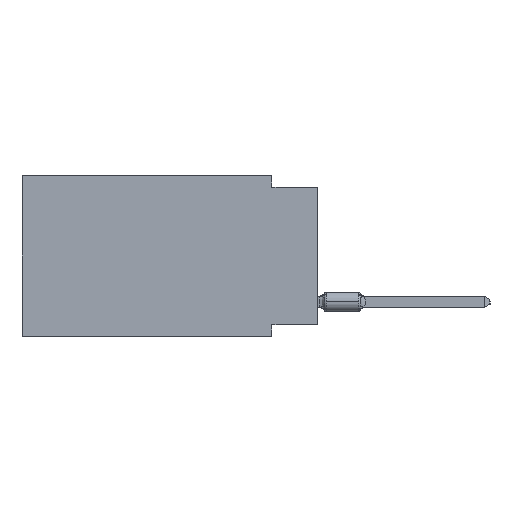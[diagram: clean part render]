
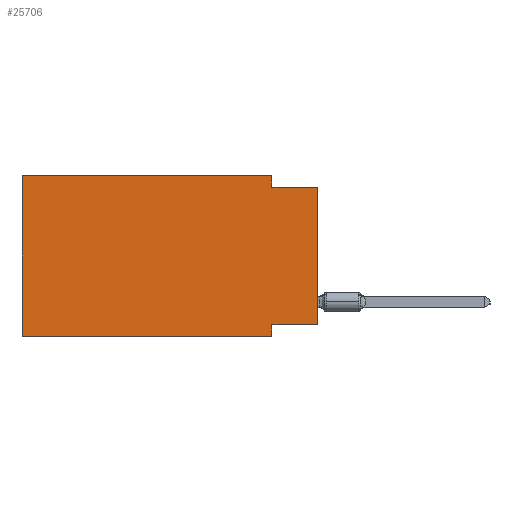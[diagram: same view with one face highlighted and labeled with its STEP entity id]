
A CAD part, left-side view. The second image highlights one B-rep face of the part: STEP entity #25706.
In plain terms, the highlighted planar face has unit normal (-1, 0, 0).
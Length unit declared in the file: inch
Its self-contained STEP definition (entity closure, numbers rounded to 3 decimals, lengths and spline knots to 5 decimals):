
#427 = LINE ( 'NONE', #22968, #40723 ) ;
#480 = CARTESIAN_POINT ( 'NONE',  ( 0., 0., 0. ) ) ;
#829 = CARTESIAN_POINT ( 'NONE',  ( 0., 0.1, -0.325 ) ) ;
#1499 = CARTESIAN_POINT ( 'NONE',  ( 0., 0.645, -0.35 ) ) ;
#3735 = VERTEX_POINT ( 'NONE', #37283 ) ;
#3793 = DIRECTION ( 'NONE',  ( 0., 0., -1. ) ) ;
#5903 = EDGE_LOOP ( 'NONE', ( #18458, #46831, #11826, #51869, #16106, #41703, #51386, #30018 ) ) ;
#9258 = EDGE_CURVE ( 'NONE', #3735, #48961, #50256, .T. ) ;
#9440 = CARTESIAN_POINT ( 'NONE',  ( 0., 0., -0.325 ) ) ;
#11186 = VERTEX_POINT ( 'NONE', #29794 ) ;
#11826 = ORIENTED_EDGE ( 'NONE', *, *, #31525, .F. ) ;
#12261 = VERTEX_POINT ( 'NONE', #15886 ) ;
#12708 = AXIS2_PLACEMENT_3D ( 'NONE', #37321, #29233, #3793 ) ;
#12890 = VECTOR ( 'NONE', #30573, 39.37008 ) ;
#13250 = CARTESIAN_POINT ( 'NONE',  ( 0., 0., -0.325 ) ) ;
#13911 = DIRECTION ( 'NONE',  ( 0., 1., 0. ) ) ;
#14426 = CARTESIAN_POINT ( 'NONE',  ( 0., 0.645, 0. ) ) ;
#15019 = VERTEX_POINT ( 'NONE', #829 ) ;
#15886 = CARTESIAN_POINT ( 'NONE',  ( 0., 0.1, -0.025 ) ) ;
#16106 = ORIENTED_EDGE ( 'NONE', *, *, #9258, .F. ) ;
#16855 = LINE ( 'NONE', #51753, #23512 ) ;
#18458 = ORIENTED_EDGE ( 'NONE', *, *, #33916, .T. ) ;
#18889 = VECTOR ( 'NONE', #29590, 39.37008 ) ;
#21222 = CARTESIAN_POINT ( 'NONE',  ( 0., 0.645, 0. ) ) ;
#21437 = LINE ( 'NONE', #480, #50778 ) ;
#22968 = CARTESIAN_POINT ( 'NONE',  ( 0., 0.1, -0.35 ) ) ;
#23324 = EDGE_CURVE ( 'NONE', #3735, #39051, #47315, .T. ) ;
#23326 = VERTEX_POINT ( 'NONE', #13250 ) ;
#23512 = VECTOR ( 'NONE', #25236, 39.37008 ) ;
#24323 = CARTESIAN_POINT ( 'NONE',  ( 0., 0.1, 0. ) ) ;
#25138 = DIRECTION ( 'NONE',  ( 0., -1., 0. ) ) ;
#25236 = DIRECTION ( 'NONE',  ( 0., -1., 0. ) ) ;
#25351 = DIRECTION ( 'NONE',  ( 0., 0., 1. ) ) ;
#25706 = ADVANCED_FACE ( 'NONE', ( #45425 ), #33417, .F. ) ;
#26791 = CARTESIAN_POINT ( 'NONE',  ( 0., 0.1, -0.35 ) ) ;
#28431 = VECTOR ( 'NONE', #30901, 39.37008 ) ;
#29233 = DIRECTION ( 'NONE',  ( 1., 0., 0. ) ) ;
#29333 = CARTESIAN_POINT ( 'NONE',  ( 0., 0., -0.025 ) ) ;
#29590 = DIRECTION ( 'NONE',  ( 0., 0., 1. ) ) ;
#29794 = CARTESIAN_POINT ( 'NONE',  ( 0., 0., -0.025 ) ) ;
#30018 = ORIENTED_EDGE ( 'NONE', *, *, #45819, .F. ) ;
#30573 = DIRECTION ( 'NONE',  ( 0., -1., 0. ) ) ;
#30684 = VERTEX_POINT ( 'NONE', #24323 ) ;
#30686 = LINE ( 'NONE', #9440, #41081 ) ;
#30901 = DIRECTION ( 'NONE',  ( 0., 0., -1. ) ) ;
#31160 = CARTESIAN_POINT ( 'NONE',  ( 0., 0.1, 0. ) ) ;
#31525 = EDGE_CURVE ( 'NONE', #30684, #12261, #40081, .T. ) ;
#33417 = PLANE ( 'NONE',  #12708 ) ;
#33916 = EDGE_CURVE ( 'NONE', #23326, #11186, #21437, .T. ) ;
#34504 = DIRECTION ( 'NONE',  ( 0., 0., -1. ) ) ;
#37283 = CARTESIAN_POINT ( 'NONE',  ( 0., 0.645, -0.35 ) ) ;
#37321 = CARTESIAN_POINT ( 'NONE',  ( 0., 0.645, 0. ) ) ;
#38952 = EDGE_CURVE ( 'NONE', #12261, #11186, #45808, .T. ) ;
#39051 = VERTEX_POINT ( 'NONE', #26791 ) ;
#40081 = LINE ( 'NONE', #31160, #28431 ) ;
#40723 = VECTOR ( 'NONE', #34504, 39.37008 ) ;
#41081 = VECTOR ( 'NONE', #13911, 39.37008 ) ;
#41703 = ORIENTED_EDGE ( 'NONE', *, *, #23324, .T. ) ;
#44849 = VECTOR ( 'NONE', #25138, 39.37008 ) ;
#45425 = FACE_OUTER_BOUND ( 'NONE', #5903, .T. ) ;
#45808 = LINE ( 'NONE', #29333, #44849 ) ;
#45819 = EDGE_CURVE ( 'NONE', #23326, #15019, #30686, .T. ) ;
#46831 = ORIENTED_EDGE ( 'NONE', *, *, #38952, .F. ) ;
#47315 = LINE ( 'NONE', #1499, #12890 ) ;
#48961 = VERTEX_POINT ( 'NONE', #14426 ) ;
#50256 = LINE ( 'NONE', #21222, #18889 ) ;
#50778 = VECTOR ( 'NONE', #25351, 39.37008 ) ;
#51386 = ORIENTED_EDGE ( 'NONE', *, *, #55075, .F. ) ;
#51576 = EDGE_CURVE ( 'NONE', #48961, #30684, #16855, .T. ) ;
#51753 = CARTESIAN_POINT ( 'NONE',  ( 0., 0.645, 0. ) ) ;
#51869 = ORIENTED_EDGE ( 'NONE', *, *, #51576, .F. ) ;
#55075 = EDGE_CURVE ( 'NONE', #15019, #39051, #427, .T. ) ;
